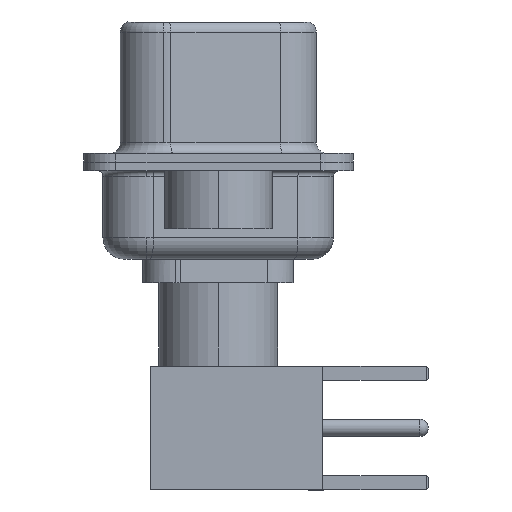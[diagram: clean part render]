
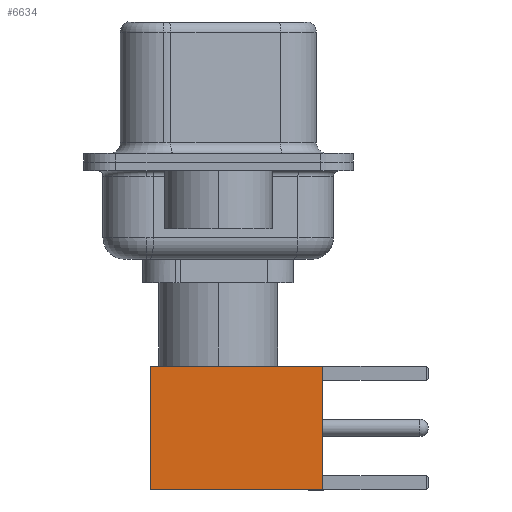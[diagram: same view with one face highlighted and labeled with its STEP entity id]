
A CAD part, left-side view. The second image highlights one B-rep face of the part: STEP entity #6634.
In plain terms, the highlighted face is planar.
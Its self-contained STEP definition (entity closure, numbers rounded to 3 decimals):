
#1651 = DIRECTION ( 'NONE',  ( 0., 1., 0. ) ) ;
#3765 = VERTEX_POINT ( 'NONE', #6218 ) ;
#3984 = CARTESIAN_POINT ( 'NONE',  ( 0., 2.875, 8. ) ) ;
#4163 = AXIS2_PLACEMENT_3D ( 'NONE', #13416, #1651, #17506 ) ;
#4251 = VECTOR ( 'NONE', #14773, 1000. ) ;
#4453 = VERTEX_POINT ( 'NONE', #12023 ) ;
#4899 = EDGE_LOOP ( 'NONE', ( #12985, #8290, #11530, #9635 ) ) ;
#5157 = VERTEX_POINT ( 'NONE', #9581 ) ;
#5338 = VECTOR ( 'NONE', #17082, 1000. ) ;
#5450 = FACE_OUTER_BOUND ( 'NONE', #4899, .T. ) ;
#6218 = CARTESIAN_POINT ( 'NONE',  ( 2.875, 2.875, 0. ) ) ;
#6285 = CARTESIAN_POINT ( 'NONE',  ( 2.875, 2.875, 0. ) ) ;
#6634 = ADVANCED_FACE ( 'NONE', ( #5450 ), #16257, .T. ) ;
#7953 = EDGE_CURVE ( 'NONE', #3765, #4453, #13459, .T. ) ;
#8220 = LINE ( 'NONE', #9446, #4251 ) ;
#8266 = VERTEX_POINT ( 'NONE', #11757 ) ;
#8290 = ORIENTED_EDGE ( 'NONE', *, *, #7953, .T. ) ;
#8368 = EDGE_CURVE ( 'NONE', #5157, #3765, #12818, .T. ) ;
#9382 = DIRECTION ( 'NONE',  ( -1., 0., 0. ) ) ;
#9446 = CARTESIAN_POINT ( 'NONE',  ( -2.875, 2.875, 0. ) ) ;
#9581 = CARTESIAN_POINT ( 'NONE',  ( 2.875, 2.875, 8. ) ) ;
#9635 = ORIENTED_EDGE ( 'NONE', *, *, #9816, .F. ) ;
#9816 = EDGE_CURVE ( 'NONE', #5157, #8266, #16022, .T. ) ;
#9854 = EDGE_CURVE ( 'NONE', #8266, #4453, #8220, .T. ) ;
#11530 = ORIENTED_EDGE ( 'NONE', *, *, #9854, .F. ) ;
#11757 = CARTESIAN_POINT ( 'NONE',  ( -2.875, 2.875, 8. ) ) ;
#12023 = CARTESIAN_POINT ( 'NONE',  ( -2.875, 2.875, 0. ) ) ;
#12029 = DIRECTION ( 'NONE',  ( -1., 0., 0. ) ) ;
#12818 = LINE ( 'NONE', #6285, #5338 ) ;
#12985 = ORIENTED_EDGE ( 'NONE', *, *, #8368, .T. ) ;
#13416 = CARTESIAN_POINT ( 'NONE',  ( 2.875, 2.875, 0. ) ) ;
#13459 = LINE ( 'NONE', #16040, #15768 ) ;
#13562 = VECTOR ( 'NONE', #12029, 1000. ) ;
#14773 = DIRECTION ( 'NONE',  ( 0., 0., -1. ) ) ;
#15768 = VECTOR ( 'NONE', #9382, 1000. ) ;
#16022 = LINE ( 'NONE', #3984, #13562 ) ;
#16040 = CARTESIAN_POINT ( 'NONE',  ( 0., 2.875, 0. ) ) ;
#16257 = PLANE ( 'NONE',  #4163 ) ;
#17082 = DIRECTION ( 'NONE',  ( 0., 0., -1. ) ) ;
#17506 = DIRECTION ( 'NONE',  ( 0., 0., 1. ) ) ;
